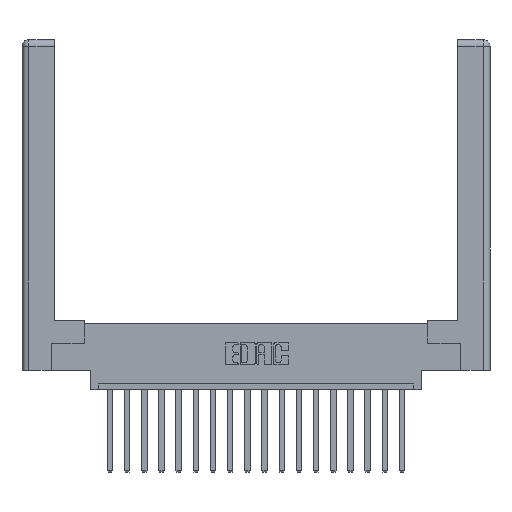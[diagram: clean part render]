
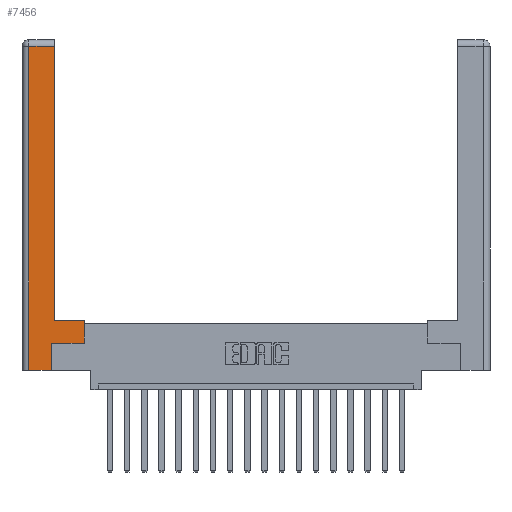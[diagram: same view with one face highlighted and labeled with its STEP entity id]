
A CAD part, top view. The second image highlights one B-rep face of the part: STEP entity #7456.
In plain terms, the highlighted planar face has unit normal (0, 0, 1).
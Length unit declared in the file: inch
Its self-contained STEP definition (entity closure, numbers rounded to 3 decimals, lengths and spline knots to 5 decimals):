
#32 = VECTOR ( 'NONE', #2422, 39.37008 ) ;
#388 = LINE ( 'NONE', #12948, #18546 ) ;
#608 = CARTESIAN_POINT ( 'NONE',  ( 0.0615, 2.94, 0. ) ) ;
#1747 = VERTEX_POINT ( 'NONE', #9886 ) ;
#1925 = LINE ( 'NONE', #12340, #4703 ) ;
#2168 = VECTOR ( 'NONE', #11082, 39.37008 ) ;
#2422 = DIRECTION ( 'NONE',  ( 0., -1., 0. ) ) ;
#2889 = LINE ( 'NONE', #15667, #11659 ) ;
#2895 = DIRECTION ( 'NONE',  ( -1., 0., 0. ) ) ;
#3056 = VERTEX_POINT ( 'NONE', #15115 ) ;
#3681 = DIRECTION ( 'NONE',  ( 1., 0., 0. ) ) ;
#4176 = ORIENTED_EDGE ( 'NONE', *, *, #15343, .T. ) ;
#4703 = VECTOR ( 'NONE', #15277, 39.37008 ) ;
#4871 = ORIENTED_EDGE ( 'NONE', *, *, #7125, .T. ) ;
#5781 = CARTESIAN_POINT ( 'NONE',  ( 0.0615, 2.94, 0. ) ) ;
#6183 = LINE ( 'NONE', #11218, #13109 ) ;
#6294 = VERTEX_POINT ( 'NONE', #11275 ) ;
#6723 = CARTESIAN_POINT ( 'NONE',  ( 0.565, 0.45, 0. ) ) ;
#6835 = VECTOR ( 'NONE', #2895, 39.37008 ) ;
#7125 = EDGE_CURVE ( 'NONE', #14991, #8766, #2889, .T. ) ;
#7456 = ADVANCED_FACE ( 'NONE', ( #12549 ), #13408, .F. ) ;
#7570 = CARTESIAN_POINT ( 'NONE',  ( 0., 0., 0. ) ) ;
#7591 = EDGE_CURVE ( 'NONE', #9375, #1747, #16013, .T. ) ;
#8388 = VECTOR ( 'NONE', #12086, 39.37008 ) ;
#8766 = VERTEX_POINT ( 'NONE', #6723 ) ;
#9375 = VERTEX_POINT ( 'NONE', #9859 ) ;
#9859 = CARTESIAN_POINT ( 'NONE',  ( 0.265, 0., 0. ) ) ;
#9862 = LINE ( 'NONE', #5781, #6835 ) ;
#9886 = CARTESIAN_POINT ( 'NONE',  ( 0.265, 0.245, 0. ) ) ;
#10077 = VERTEX_POINT ( 'NONE', #18755 ) ;
#11031 = DIRECTION ( 'NONE',  ( 0., 1., 0. ) ) ;
#11058 = ORIENTED_EDGE ( 'NONE', *, *, #12952, .T. ) ;
#11082 = DIRECTION ( 'NONE',  ( 0., 1., 0. ) ) ;
#11218 = CARTESIAN_POINT ( 'NONE',  ( 0.565, 0.245, 0. ) ) ;
#11275 = CARTESIAN_POINT ( 'NONE',  ( 0.0615, 0., 0. ) ) ;
#11301 = ORIENTED_EDGE ( 'NONE', *, *, #12592, .T. ) ;
#11323 = CARTESIAN_POINT ( 'NONE',  ( 0.0615, 0., 0. ) ) ;
#11659 = VECTOR ( 'NONE', #11031, 39.37008 ) ;
#12084 = CARTESIAN_POINT ( 'NONE',  ( 0.565, 0.245, 0. ) ) ;
#12086 = DIRECTION ( 'NONE',  ( 0., 1., 0. ) ) ;
#12340 = CARTESIAN_POINT ( 'NONE',  ( 0.295, 0.45, 0. ) ) ;
#12543 = ORIENTED_EDGE ( 'NONE', *, *, #15030, .T. ) ;
#12549 = FACE_OUTER_BOUND ( 'NONE', #18573, .T. ) ;
#12592 = EDGE_CURVE ( 'NONE', #10077, #17006, #9862, .T. ) ;
#12691 = ORIENTED_EDGE ( 'NONE', *, *, #7591, .T. ) ;
#12948 = CARTESIAN_POINT ( 'NONE',  ( 0.265, 0., 0. ) ) ;
#12952 = EDGE_CURVE ( 'NONE', #6294, #9375, #388, .T. ) ;
#13109 = VECTOR ( 'NONE', #3681, 39.37008 ) ;
#13408 = PLANE ( 'NONE',  #17482 ) ;
#13986 = CARTESIAN_POINT ( 'NONE',  ( 0.265, 0.245, 0. ) ) ;
#14373 = DIRECTION ( 'NONE',  ( 1., 0., 0. ) ) ;
#14709 = DIRECTION ( 'NONE',  ( 0., 0., -1. ) ) ;
#14975 = CARTESIAN_POINT ( 'NONE',  ( 0.295, 3., 0. ) ) ;
#14991 = VERTEX_POINT ( 'NONE', #12084 ) ;
#15030 = EDGE_CURVE ( 'NONE', #8766, #3056, #1925, .T. ) ;
#15115 = CARTESIAN_POINT ( 'NONE',  ( 0.295, 0.45, 0. ) ) ;
#15277 = DIRECTION ( 'NONE',  ( -1., 0., 0. ) ) ;
#15343 = EDGE_CURVE ( 'NONE', #3056, #10077, #17596, .T. ) ;
#15667 = CARTESIAN_POINT ( 'NONE',  ( 0.565, 0.45, 0. ) ) ;
#16013 = LINE ( 'NONE', #13986, #2168 ) ;
#16188 = ORIENTED_EDGE ( 'NONE', *, *, #17579, .T. ) ;
#17006 = VERTEX_POINT ( 'NONE', #608 ) ;
#17083 = EDGE_CURVE ( 'NONE', #17006, #6294, #17573, .T. ) ;
#17482 = AXIS2_PLACEMENT_3D ( 'NONE', #7570, #14709, #17858 ) ;
#17573 = LINE ( 'NONE', #11323, #32 ) ;
#17579 = EDGE_CURVE ( 'NONE', #1747, #14991, #6183, .T. ) ;
#17596 = LINE ( 'NONE', #14975, #8388 ) ;
#17858 = DIRECTION ( 'NONE',  ( -1., 0., 0. ) ) ;
#18546 = VECTOR ( 'NONE', #14373, 39.37008 ) ;
#18573 = EDGE_LOOP ( 'NONE', ( #4176, #11301, #18688, #11058, #12691, #16188, #4871, #12543 ) ) ;
#18688 = ORIENTED_EDGE ( 'NONE', *, *, #17083, .T. ) ;
#18755 = CARTESIAN_POINT ( 'NONE',  ( 0.295, 2.94, 0. ) ) ;
